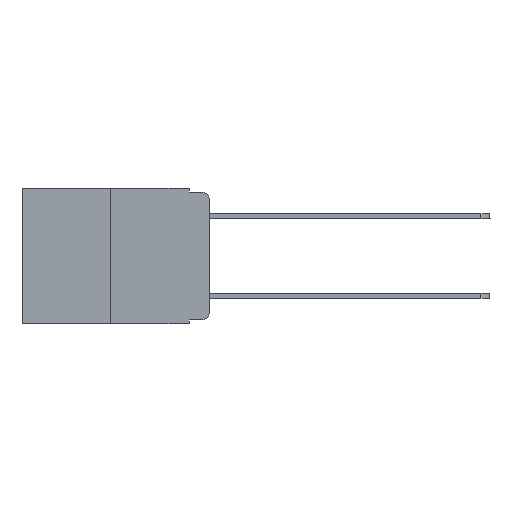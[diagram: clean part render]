
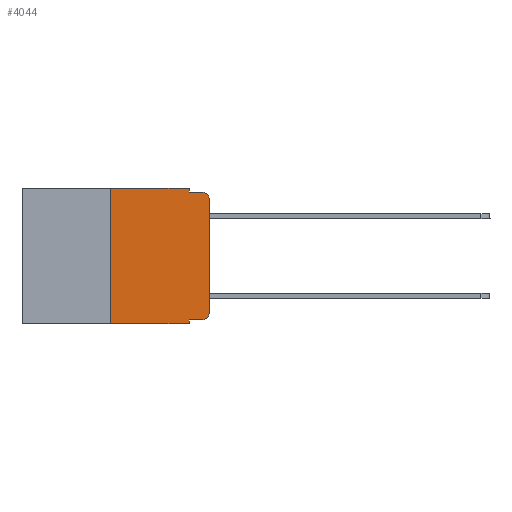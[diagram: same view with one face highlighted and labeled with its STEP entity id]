
A CAD part, left-side view. The second image highlights one B-rep face of the part: STEP entity #4044.
In plain terms, the highlighted planar face has unit normal (-1, 0, 0).
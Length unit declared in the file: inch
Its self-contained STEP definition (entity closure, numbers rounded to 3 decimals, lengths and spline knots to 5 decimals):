
#267 = LINE ( 'NONE', #1858, #5436 ) ;
#1195 = VERTEX_POINT ( 'NONE', #18481 ) ;
#1241 = EDGE_CURVE ( 'NONE', #11117, #1195, #13574, .T. ) ;
#1766 = VERTEX_POINT ( 'NONE', #12916 ) ;
#1858 = CARTESIAN_POINT ( 'NONE',  ( 0., 0.25, 0. ) ) ;
#2274 = VECTOR ( 'NONE', #17912, 39.37008 ) ;
#2278 = CARTESIAN_POINT ( 'NONE',  ( 0., 0.02, -0.333 ) ) ;
#2927 = CARTESIAN_POINT ( 'NONE',  ( 0., 0.473, -0.343 ) ) ;
#3093 = DIRECTION ( 'NONE',  ( -1., 0., 0. ) ) ;
#3357 = EDGE_CURVE ( 'NONE', #14997, #9293, #5085, .T. ) ;
#3410 = CARTESIAN_POINT ( 'NONE',  ( 0., 0.25, -0.343 ) ) ;
#3491 = DIRECTION ( 'NONE',  ( 0., 0., 1. ) ) ;
#3773 = DIRECTION ( 'NONE',  ( 0., -1., 0. ) ) ;
#3827 = CARTESIAN_POINT ( 'NONE',  ( 0., 0.051, -0.01 ) ) ;
#3873 = CARTESIAN_POINT ( 'NONE',  ( 0., 0.473, 0. ) ) ;
#4044 = ADVANCED_FACE ( 'NONE', ( #22958 ), #17921, .F. ) ;
#4680 = LINE ( 'NONE', #2927, #5899 ) ;
#4716 = VECTOR ( 'NONE', #20086, 39.37008 ) ;
#4888 = ORIENTED_EDGE ( 'NONE', *, *, #11767, .F. ) ;
#4946 = VECTOR ( 'NONE', #12690, 39.37008 ) ;
#5085 = LINE ( 'NONE', #14233, #4716 ) ;
#5203 = AXIS2_PLACEMENT_3D ( 'NONE', #19386, #3093, #10315 ) ;
#5436 = VECTOR ( 'NONE', #3491, 39.37008 ) ;
#5559 = CIRCLE ( 'NONE', #5203, 0.02 ) ;
#5606 = EDGE_CURVE ( 'NONE', #21283, #11117, #20078, .T. ) ;
#5727 = DIRECTION ( 'NONE',  ( 0., 0., 1. ) ) ;
#5843 = VERTEX_POINT ( 'NONE', #15168 ) ;
#5883 = VECTOR ( 'NONE', #21952, 39.37008 ) ;
#5899 = VECTOR ( 'NONE', #19088, 39.37008 ) ;
#6065 = DIRECTION ( 'NONE',  ( -1., 0., 0. ) ) ;
#6832 = DIRECTION ( 'NONE',  ( 0., 0., -1. ) ) ;
#7343 = LINE ( 'NONE', #10683, #4946 ) ;
#7504 = CARTESIAN_POINT ( 'NONE',  ( 0., 0., 0. ) ) ;
#7695 = EDGE_CURVE ( 'NONE', #12192, #5843, #267, .T. ) ;
#7767 = ORIENTED_EDGE ( 'NONE', *, *, #1241, .T. ) ;
#8745 = VERTEX_POINT ( 'NONE', #10617 ) ;
#8798 = CARTESIAN_POINT ( 'NONE',  ( 0., 0.051, -0.01 ) ) ;
#8947 = EDGE_CURVE ( 'NONE', #1195, #1766, #22080, .T. ) ;
#9292 = VECTOR ( 'NONE', #5727, 39.37008 ) ;
#9293 = VERTEX_POINT ( 'NONE', #8798 ) ;
#9894 = ORIENTED_EDGE ( 'NONE', *, *, #8947, .T. ) ;
#10315 = DIRECTION ( 'NONE',  ( 0., 0., -1. ) ) ;
#10419 = ORIENTED_EDGE ( 'NONE', *, *, #13537, .T. ) ;
#10617 = CARTESIAN_POINT ( 'NONE',  ( 0., 0.051, -0.343 ) ) ;
#10683 = CARTESIAN_POINT ( 'NONE',  ( 0., 0.051, 0. ) ) ;
#10767 = LINE ( 'NONE', #3873, #2274 ) ;
#10950 = EDGE_CURVE ( 'NONE', #21283, #8745, #7343, .T. ) ;
#11117 = VERTEX_POINT ( 'NONE', #2278 ) ;
#11347 = CARTESIAN_POINT ( 'NONE',  ( 0., 0.051, -0.333 ) ) ;
#11528 = DIRECTION ( 'NONE',  ( 0., 0., -1. ) ) ;
#11678 = ORIENTED_EDGE ( 'NONE', *, *, #10950, .F. ) ;
#11767 = EDGE_CURVE ( 'NONE', #9293, #12784, #21705, .T. ) ;
#12192 = VERTEX_POINT ( 'NONE', #3410 ) ;
#12450 = EDGE_CURVE ( 'NONE', #12192, #8745, #4680, .T. ) ;
#12690 = DIRECTION ( 'NONE',  ( 0., 0., -1. ) ) ;
#12784 = VERTEX_POINT ( 'NONE', #12956 ) ;
#12905 = CARTESIAN_POINT ( 'NONE',  ( 0., 0.051, 0. ) ) ;
#12916 = CARTESIAN_POINT ( 'NONE',  ( 0., 0., -0.03 ) ) ;
#12956 = CARTESIAN_POINT ( 'NONE',  ( 0., 0.02, -0.01 ) ) ;
#13537 = EDGE_CURVE ( 'NONE', #1766, #12784, #5559, .T. ) ;
#13574 = CIRCLE ( 'NONE', #16639, 0.02 ) ;
#13852 = CARTESIAN_POINT ( 'NONE',  ( 0., 0.473, 0. ) ) ;
#14093 = DIRECTION ( 'NONE',  ( 1., 0., 0. ) ) ;
#14233 = CARTESIAN_POINT ( 'NONE',  ( 0., 0.051, 0. ) ) ;
#14496 = CARTESIAN_POINT ( 'NONE',  ( 0., 0.051, -0.333 ) ) ;
#14997 = VERTEX_POINT ( 'NONE', #12905 ) ;
#15168 = CARTESIAN_POINT ( 'NONE',  ( 0., 0.25, 0. ) ) ;
#15418 = EDGE_CURVE ( 'NONE', #5843, #14997, #10767, .T. ) ;
#16011 = AXIS2_PLACEMENT_3D ( 'NONE', #13852, #14093, #6832 ) ;
#16043 = ORIENTED_EDGE ( 'NONE', *, *, #15418, .F. ) ;
#16639 = AXIS2_PLACEMENT_3D ( 'NONE', #20509, #6065, #11528 ) ;
#17912 = DIRECTION ( 'NONE',  ( 0., -1., 0. ) ) ;
#17921 = PLANE ( 'NONE',  #16011 ) ;
#18481 = CARTESIAN_POINT ( 'NONE',  ( 0., 0., -0.313 ) ) ;
#19088 = DIRECTION ( 'NONE',  ( 0., -1., 0. ) ) ;
#19295 = ORIENTED_EDGE ( 'NONE', *, *, #3357, .F. ) ;
#19386 = CARTESIAN_POINT ( 'NONE',  ( 0., 0.02, -0.03 ) ) ;
#19604 = ORIENTED_EDGE ( 'NONE', *, *, #12450, .T. ) ;
#19768 = ORIENTED_EDGE ( 'NONE', *, *, #7695, .F. ) ;
#20078 = LINE ( 'NONE', #11347, #23243 ) ;
#20086 = DIRECTION ( 'NONE',  ( 0., 0., -1. ) ) ;
#20509 = CARTESIAN_POINT ( 'NONE',  ( 0., 0.02, -0.313 ) ) ;
#21283 = VERTEX_POINT ( 'NONE', #14496 ) ;
#21705 = LINE ( 'NONE', #3827, #5883 ) ;
#21952 = DIRECTION ( 'NONE',  ( 0., -1., 0. ) ) ;
#22060 = EDGE_LOOP ( 'NONE', ( #9894, #10419, #4888, #19295, #16043, #19768, #19604, #11678, #22741, #7767 ) ) ;
#22080 = LINE ( 'NONE', #7504, #9292 ) ;
#22741 = ORIENTED_EDGE ( 'NONE', *, *, #5606, .T. ) ;
#22958 = FACE_OUTER_BOUND ( 'NONE', #22060, .T. ) ;
#23243 = VECTOR ( 'NONE', #3773, 39.37008 ) ;
